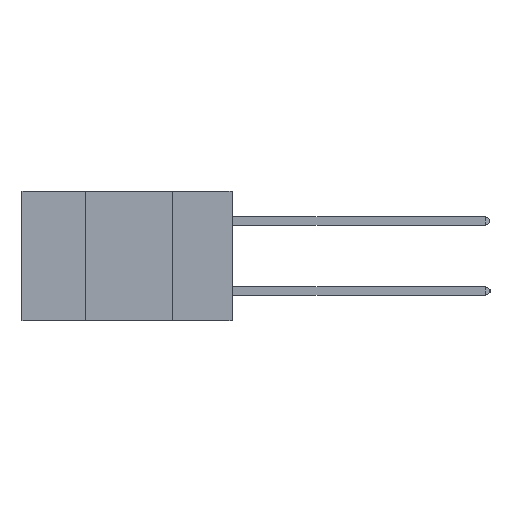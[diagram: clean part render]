
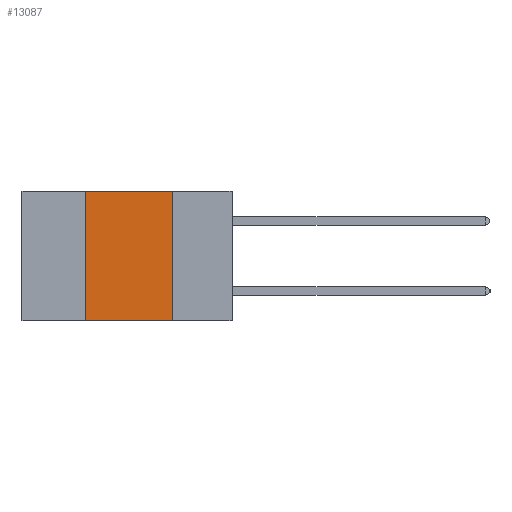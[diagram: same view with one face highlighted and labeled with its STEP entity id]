
A CAD part, left-side view. The second image highlights one B-rep face of the part: STEP entity #13087.
In plain terms, the highlighted planar face has unit normal (-1, 0, 0).
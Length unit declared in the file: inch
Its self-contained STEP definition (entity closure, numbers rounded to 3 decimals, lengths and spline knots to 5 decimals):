
#205 = EDGE_CURVE ( 'NONE', #1106, #13122, #5986, .T. ) ;
#525 = VECTOR ( 'NONE', #9421, 39.37008 ) ;
#1106 = VERTEX_POINT ( 'NONE', #11390 ) ;
#1233 = FACE_OUTER_BOUND ( 'NONE', #11115, .T. ) ;
#2006 = VERTEX_POINT ( 'NONE', #3810 ) ;
#2040 = CARTESIAN_POINT ( 'NONE',  ( 0., 0.6, 0. ) ) ;
#2147 = VECTOR ( 'NONE', #6862, 39.37008 ) ;
#2249 = CARTESIAN_POINT ( 'NONE',  ( 0., 0.17, 0. ) ) ;
#2945 = CARTESIAN_POINT ( 'NONE',  ( 0., 0.6, -0.37 ) ) ;
#2949 = ORIENTED_EDGE ( 'NONE', *, *, #7547, .F. ) ;
#3805 = EDGE_CURVE ( 'NONE', #2006, #11051, #12029, .T. ) ;
#3810 = CARTESIAN_POINT ( 'NONE',  ( 0., 0.42, -0.37 ) ) ;
#4914 = LINE ( 'NONE', #13389, #7035 ) ;
#5705 = DIRECTION ( 'NONE',  ( 0., 0., 1. ) ) ;
#5986 = LINE ( 'NONE', #11297, #11589 ) ;
#6862 = DIRECTION ( 'NONE',  ( 0., 0., -1. ) ) ;
#7035 = VECTOR ( 'NONE', #5705, 39.37008 ) ;
#7488 = EDGE_CURVE ( 'NONE', #2006, #1106, #4914, .T. ) ;
#7547 = EDGE_CURVE ( 'NONE', #13122, #11051, #10480, .T. ) ;
#8360 = DIRECTION ( 'NONE',  ( 1., 0., 0. ) ) ;
#9421 = DIRECTION ( 'NONE',  ( 0., -1., 0. ) ) ;
#9425 = DIRECTION ( 'NONE',  ( 0., 0., -1. ) ) ;
#10194 = ORIENTED_EDGE ( 'NONE', *, *, #3805, .T. ) ;
#10355 = PLANE ( 'NONE',  #12561 ) ;
#10480 = LINE ( 'NONE', #11131, #2147 ) ;
#11051 = VERTEX_POINT ( 'NONE', #12274 ) ;
#11115 = EDGE_LOOP ( 'NONE', ( #2949, #12933, #12086, #10194 ) ) ;
#11131 = CARTESIAN_POINT ( 'NONE',  ( 0., 0.17, 0. ) ) ;
#11297 = CARTESIAN_POINT ( 'NONE',  ( 0., 0.6, 0. ) ) ;
#11390 = CARTESIAN_POINT ( 'NONE',  ( 0., 0.42, 0. ) ) ;
#11589 = VECTOR ( 'NONE', #13493, 39.37008 ) ;
#12029 = LINE ( 'NONE', #2945, #525 ) ;
#12086 = ORIENTED_EDGE ( 'NONE', *, *, #7488, .F. ) ;
#12274 = CARTESIAN_POINT ( 'NONE',  ( 0., 0.17, -0.37 ) ) ;
#12561 = AXIS2_PLACEMENT_3D ( 'NONE', #2040, #8360, #9425 ) ;
#12933 = ORIENTED_EDGE ( 'NONE', *, *, #205, .F. ) ;
#13087 = ADVANCED_FACE ( 'NONE', ( #1233 ), #10355, .F. ) ;
#13122 = VERTEX_POINT ( 'NONE', #2249 ) ;
#13389 = CARTESIAN_POINT ( 'NONE',  ( 0., 0.42, 0. ) ) ;
#13493 = DIRECTION ( 'NONE',  ( 0., -1., 0. ) ) ;
